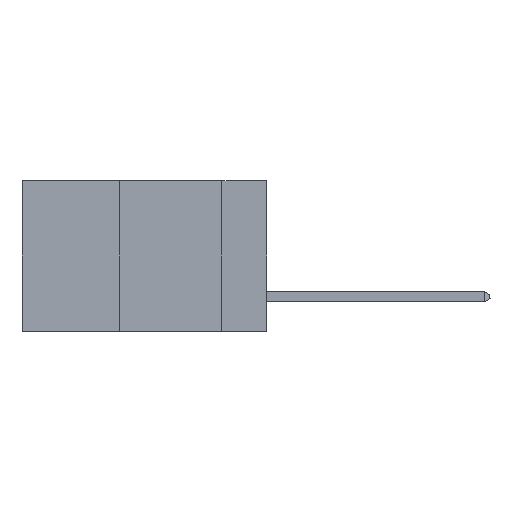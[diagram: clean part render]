
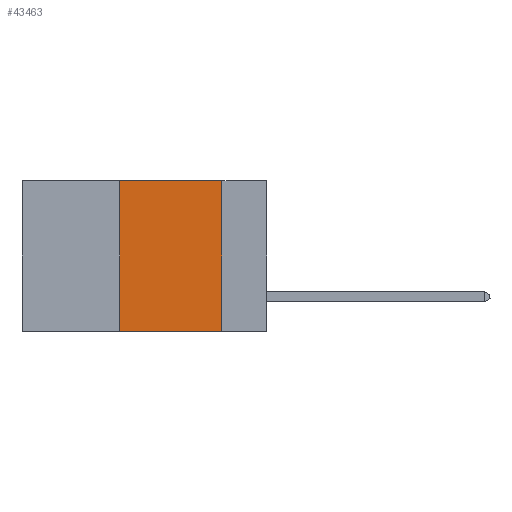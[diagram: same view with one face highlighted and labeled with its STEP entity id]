
A CAD part, left-side view. The second image highlights one B-rep face of the part: STEP entity #43463.
In plain terms, the highlighted planar face has unit normal (-1, 0, 0).
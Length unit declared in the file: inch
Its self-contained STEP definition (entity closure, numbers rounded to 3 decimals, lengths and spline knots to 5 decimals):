
#2383 = PLANE ( 'NONE',  #41240 ) ;
#4418 = CARTESIAN_POINT ( 'NONE',  ( 0., 0.36, 0. ) ) ;
#6560 = VECTOR ( 'NONE', #14489, 39.37008 ) ;
#8190 = EDGE_LOOP ( 'NONE', ( #38999, #36132, #18793, #47107 ) ) ;
#10192 = FACE_OUTER_BOUND ( 'NONE', #8190, .T. ) ;
#10821 = CARTESIAN_POINT ( 'NONE',  ( 0., 0.36, -0.37 ) ) ;
#13272 = LINE ( 'NONE', #18490, #37022 ) ;
#13413 = CARTESIAN_POINT ( 'NONE',  ( 0., 0.6, 0. ) ) ;
#14489 = DIRECTION ( 'NONE',  ( 0., 0., -1. ) ) ;
#17104 = CARTESIAN_POINT ( 'NONE',  ( 0., 0.6, 0. ) ) ;
#17429 = CARTESIAN_POINT ( 'NONE',  ( 0., 0.11, -0.37 ) ) ;
#18490 = CARTESIAN_POINT ( 'NONE',  ( 0., 0.6, -0.37 ) ) ;
#18793 = ORIENTED_EDGE ( 'NONE', *, *, #43254, .F. ) ;
#18995 = VERTEX_POINT ( 'NONE', #29869 ) ;
#19758 = EDGE_CURVE ( 'NONE', #23950, #41746, #13272, .T. ) ;
#21595 = CARTESIAN_POINT ( 'NONE',  ( 0., 0.11, 0. ) ) ;
#23059 = CARTESIAN_POINT ( 'NONE',  ( 0., 0.11, 0. ) ) ;
#23950 = VERTEX_POINT ( 'NONE', #10821 ) ;
#24923 = LINE ( 'NONE', #21595, #6560 ) ;
#25093 = DIRECTION ( 'NONE',  ( 0., 0., -1. ) ) ;
#26164 = DIRECTION ( 'NONE',  ( 0., -1., 0. ) ) ;
#27362 = EDGE_CURVE ( 'NONE', #37826, #41746, #24923, .T. ) ;
#28060 = LINE ( 'NONE', #13413, #39884 ) ;
#28751 = DIRECTION ( 'NONE',  ( 1., 0., 0. ) ) ;
#29869 = CARTESIAN_POINT ( 'NONE',  ( 0., 0.36, 0. ) ) ;
#34744 = DIRECTION ( 'NONE',  ( 0., 0., 1. ) ) ;
#36132 = ORIENTED_EDGE ( 'NONE', *, *, #42254, .F. ) ;
#37022 = VECTOR ( 'NONE', #26164, 39.37008 ) ;
#37428 = LINE ( 'NONE', #4418, #42774 ) ;
#37826 = VERTEX_POINT ( 'NONE', #23059 ) ;
#38999 = ORIENTED_EDGE ( 'NONE', *, *, #27362, .F. ) ;
#39449 = DIRECTION ( 'NONE',  ( 0., -1., 0. ) ) ;
#39884 = VECTOR ( 'NONE', #39449, 39.37008 ) ;
#41240 = AXIS2_PLACEMENT_3D ( 'NONE', #17104, #28751, #25093 ) ;
#41746 = VERTEX_POINT ( 'NONE', #17429 ) ;
#42254 = EDGE_CURVE ( 'NONE', #18995, #37826, #28060, .T. ) ;
#42774 = VECTOR ( 'NONE', #34744, 39.37008 ) ;
#43254 = EDGE_CURVE ( 'NONE', #23950, #18995, #37428, .T. ) ;
#43463 = ADVANCED_FACE ( 'NONE', ( #10192 ), #2383, .F. ) ;
#47107 = ORIENTED_EDGE ( 'NONE', *, *, #19758, .T. ) ;
